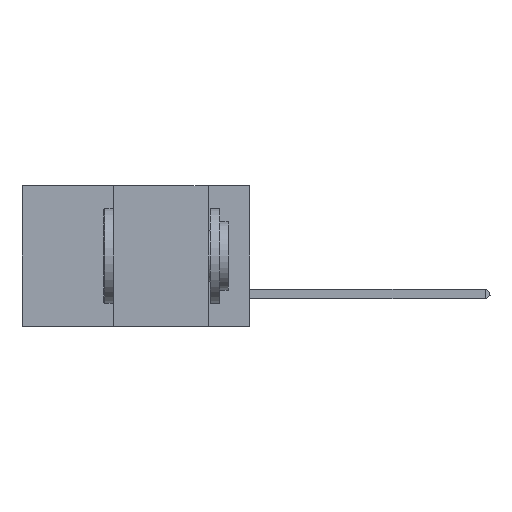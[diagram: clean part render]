
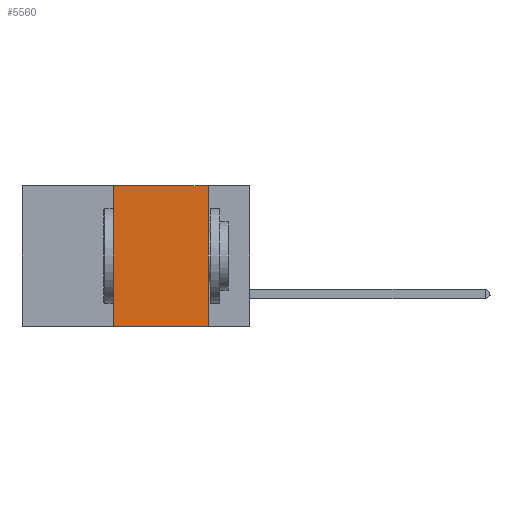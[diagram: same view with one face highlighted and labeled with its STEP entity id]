
A CAD part, left-side view. The second image highlights one B-rep face of the part: STEP entity #5560.
In plain terms, the highlighted planar face has unit normal (-1, 0, 0).
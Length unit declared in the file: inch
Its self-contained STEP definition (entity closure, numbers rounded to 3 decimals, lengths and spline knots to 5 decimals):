
#925 = EDGE_CURVE ( 'NONE', #13049, #12624, #19284, .T. ) ;
#1629 = ORIENTED_EDGE ( 'NONE', *, *, #925, .T. ) ;
#2847 = CARTESIAN_POINT ( 'NONE',  ( 0., 0.11, 0. ) ) ;
#3012 = DIRECTION ( 'NONE',  ( 0., 0., -1. ) ) ;
#4206 = CARTESIAN_POINT ( 'NONE',  ( 0., 0.36, 0. ) ) ;
#4375 = EDGE_CURVE ( 'NONE', #20189, #7947, #13551, .T. ) ;
#4545 = CARTESIAN_POINT ( 'NONE',  ( 0., 0.36, -0.37 ) ) ;
#4987 = CARTESIAN_POINT ( 'NONE',  ( 0., 0.6, 0. ) ) ;
#5560 = ADVANCED_FACE ( 'NONE', ( #22524 ), #10210, .F. ) ;
#6209 = ORIENTED_EDGE ( 'NONE', *, *, #17925, .F. ) ;
#7947 = VERTEX_POINT ( 'NONE', #2847 ) ;
#8344 = ORIENTED_EDGE ( 'NONE', *, *, #12027, .F. ) ;
#8478 = DIRECTION ( 'NONE',  ( 0., 0., -1. ) ) ;
#9264 = LINE ( 'NONE', #13398, #20211 ) ;
#9515 = DIRECTION ( 'NONE',  ( 0., -1., 0. ) ) ;
#10210 = PLANE ( 'NONE',  #12438 ) ;
#10687 = LINE ( 'NONE', #4206, #21910 ) ;
#12022 = CARTESIAN_POINT ( 'NONE',  ( 0., 0.36, 0. ) ) ;
#12027 = EDGE_CURVE ( 'NONE', #13049, #20189, #10687, .T. ) ;
#12234 = DIRECTION ( 'NONE',  ( 0., -1., 0. ) ) ;
#12438 = AXIS2_PLACEMENT_3D ( 'NONE', #4987, #22439, #8478 ) ;
#12519 = CARTESIAN_POINT ( 'NONE',  ( 0., 0.6, 0. ) ) ;
#12624 = VERTEX_POINT ( 'NONE', #17137 ) ;
#13049 = VERTEX_POINT ( 'NONE', #4545 ) ;
#13295 = DIRECTION ( 'NONE',  ( 0., 0., 1. ) ) ;
#13398 = CARTESIAN_POINT ( 'NONE',  ( 0., 0.11, 0. ) ) ;
#13551 = LINE ( 'NONE', #12519, #14669 ) ;
#14669 = VECTOR ( 'NONE', #12234, 39.37008 ) ;
#15195 = VECTOR ( 'NONE', #9515, 39.37008 ) ;
#17137 = CARTESIAN_POINT ( 'NONE',  ( 0., 0.11, -0.37 ) ) ;
#17925 = EDGE_CURVE ( 'NONE', #7947, #12624, #9264, .T. ) ;
#19284 = LINE ( 'NONE', #21373, #15195 ) ;
#20189 = VERTEX_POINT ( 'NONE', #12022 ) ;
#20211 = VECTOR ( 'NONE', #3012, 39.37008 ) ;
#21373 = CARTESIAN_POINT ( 'NONE',  ( 0., 0.6, -0.37 ) ) ;
#21910 = VECTOR ( 'NONE', #13295, 39.37008 ) ;
#22123 = ORIENTED_EDGE ( 'NONE', *, *, #4375, .F. ) ;
#22439 = DIRECTION ( 'NONE',  ( 1., 0., 0. ) ) ;
#22488 = EDGE_LOOP ( 'NONE', ( #6209, #22123, #8344, #1629 ) ) ;
#22524 = FACE_OUTER_BOUND ( 'NONE', #22488, .T. ) ;
